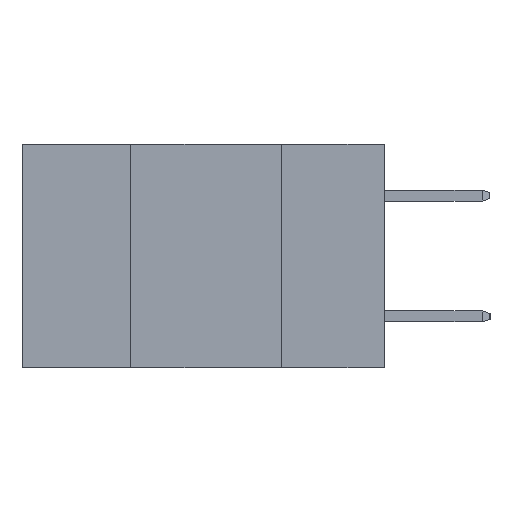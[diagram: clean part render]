
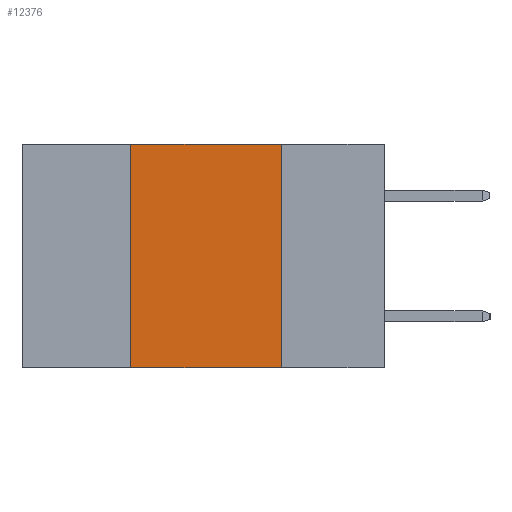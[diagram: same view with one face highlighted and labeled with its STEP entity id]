
A CAD part, left-side view. The second image highlights one B-rep face of the part: STEP entity #12376.
In plain terms, the highlighted planar face has unit normal (-1, 0, 0).
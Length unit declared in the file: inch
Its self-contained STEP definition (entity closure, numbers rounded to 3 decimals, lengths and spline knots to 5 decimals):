
#159 = CARTESIAN_POINT ( 'NONE',  ( 0., 0.42, -0.37 ) ) ;
#350 = DIRECTION ( 'NONE',  ( 1., 0., 0. ) ) ;
#359 = LINE ( 'NONE', #7438, #10524 ) ;
#480 = CARTESIAN_POINT ( 'NONE',  ( 0., 0.17, 0. ) ) ;
#1659 = CARTESIAN_POINT ( 'NONE',  ( 0., 0.6, 0. ) ) ;
#2298 = LINE ( 'NONE', #13396, #15822 ) ;
#2566 = VECTOR ( 'NONE', #8132, 39.37008 ) ;
#3004 = AXIS2_PLACEMENT_3D ( 'NONE', #1659, #350, #9639 ) ;
#3298 = ORIENTED_EDGE ( 'NONE', *, *, #15164, .F. ) ;
#3350 = LINE ( 'NONE', #7315, #16799 ) ;
#3724 = ORIENTED_EDGE ( 'NONE', *, *, #8693, .F. ) ;
#4152 = VERTEX_POINT ( 'NONE', #4529 ) ;
#4529 = CARTESIAN_POINT ( 'NONE',  ( 0., 0.42, 0. ) ) ;
#5128 = CARTESIAN_POINT ( 'NONE',  ( 0., 0.17, -0.37 ) ) ;
#5856 = VERTEX_POINT ( 'NONE', #9906 ) ;
#6008 = EDGE_CURVE ( 'NONE', #5856, #10843, #3350, .T. ) ;
#6486 = FACE_OUTER_BOUND ( 'NONE', #13850, .T. ) ;
#6974 = PLANE ( 'NONE',  #3004 ) ;
#7227 = EDGE_CURVE ( 'NONE', #5856, #4152, #16080, .T. ) ;
#7315 = CARTESIAN_POINT ( 'NONE',  ( 0., 0.6, -0.37 ) ) ;
#7352 = DIRECTION ( 'NONE',  ( 0., -1., 0. ) ) ;
#7438 = CARTESIAN_POINT ( 'NONE',  ( 0., 0.17, -0.37 ) ) ;
#8132 = DIRECTION ( 'NONE',  ( 0., 0., 1. ) ) ;
#8693 = EDGE_CURVE ( 'NONE', #4152, #8793, #2298, .T. ) ;
#8793 = VERTEX_POINT ( 'NONE', #480 ) ;
#9639 = DIRECTION ( 'NONE',  ( 0., 0., -1. ) ) ;
#9906 = CARTESIAN_POINT ( 'NONE',  ( 0., 0.42, -0.37 ) ) ;
#10186 = DIRECTION ( 'NONE',  ( 0., 0., -1. ) ) ;
#10524 = VECTOR ( 'NONE', #10186, 39.37008 ) ;
#10843 = VERTEX_POINT ( 'NONE', #5128 ) ;
#11145 = ORIENTED_EDGE ( 'NONE', *, *, #7227, .F. ) ;
#11538 = ORIENTED_EDGE ( 'NONE', *, *, #6008, .T. ) ;
#12376 = ADVANCED_FACE ( 'NONE', ( #6486 ), #6974, .F. ) ;
#13396 = CARTESIAN_POINT ( 'NONE',  ( 0., 0.6, 0. ) ) ;
#13850 = EDGE_LOOP ( 'NONE', ( #3298, #3724, #11145, #11538 ) ) ;
#14751 = DIRECTION ( 'NONE',  ( 0., -1., 0. ) ) ;
#15164 = EDGE_CURVE ( 'NONE', #8793, #10843, #359, .T. ) ;
#15822 = VECTOR ( 'NONE', #14751, 39.37008 ) ;
#16080 = LINE ( 'NONE', #159, #2566 ) ;
#16799 = VECTOR ( 'NONE', #7352, 39.37008 ) ;
